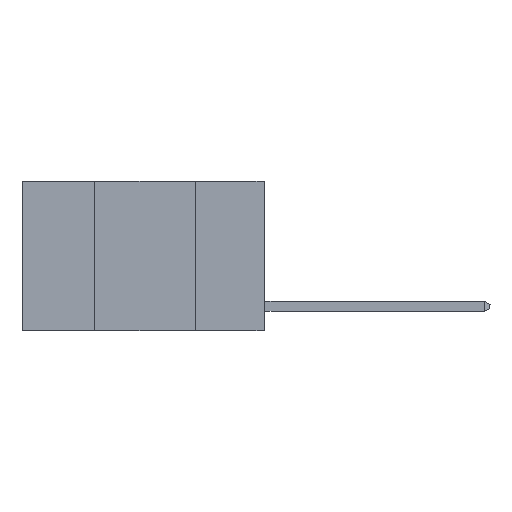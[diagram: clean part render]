
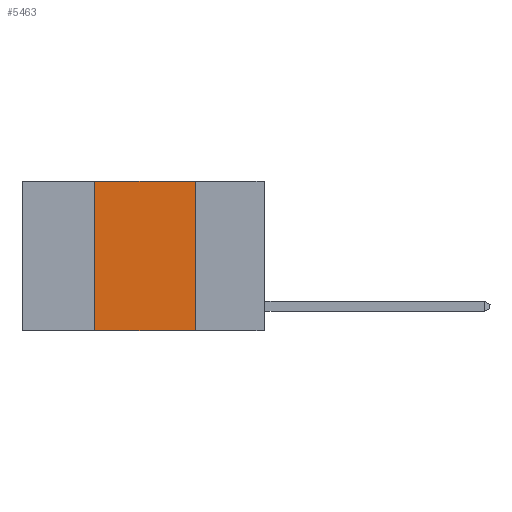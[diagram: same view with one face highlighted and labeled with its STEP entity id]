
A CAD part, left-side view. The second image highlights one B-rep face of the part: STEP entity #5463.
In plain terms, the highlighted planar face has unit normal (-1, 0, 0).
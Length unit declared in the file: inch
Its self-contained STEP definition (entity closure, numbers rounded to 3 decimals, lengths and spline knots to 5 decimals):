
#234 = LINE ( 'NONE', #14729, #4201 ) ;
#480 = AXIS2_PLACEMENT_3D ( 'NONE', #19061, #17314, #17523 ) ;
#2029 = VERTEX_POINT ( 'NONE', #8296 ) ;
#2222 = DIRECTION ( 'NONE',  ( 0., -1., 0. ) ) ;
#3056 = PLANE ( 'NONE',  #480 ) ;
#3435 = CARTESIAN_POINT ( 'NONE',  ( 0., 0.6, 0. ) ) ;
#3631 = VECTOR ( 'NONE', #7467, 39.37008 ) ;
#4201 = VECTOR ( 'NONE', #19261, 39.37008 ) ;
#4958 = EDGE_CURVE ( 'NONE', #5296, #2029, #12539, .T. ) ;
#5296 = VERTEX_POINT ( 'NONE', #13545 ) ;
#5312 = EDGE_CURVE ( 'NONE', #13542, #7009, #18152, .T. ) ;
#5463 = ADVANCED_FACE ( 'NONE', ( #18385 ), #3056, .F. ) ;
#6445 = EDGE_LOOP ( 'NONE', ( #18474, #13665, #19468, #19474 ) ) ;
#7009 = VERTEX_POINT ( 'NONE', #13013 ) ;
#7467 = DIRECTION ( 'NONE',  ( 0., 0., -1. ) ) ;
#8296 = CARTESIAN_POINT ( 'NONE',  ( 0., 0.42, 0. ) ) ;
#9358 = CARTESIAN_POINT ( 'NONE',  ( 0., 0.17, 0. ) ) ;
#10073 = EDGE_CURVE ( 'NONE', #2029, #13542, #19752, .T. ) ;
#10700 = CARTESIAN_POINT ( 'NONE',  ( 0., 0.42, 0. ) ) ;
#12539 = LINE ( 'NONE', #10700, #12769 ) ;
#12769 = VECTOR ( 'NONE', #13976, 39.37008 ) ;
#13013 = CARTESIAN_POINT ( 'NONE',  ( 0., 0.17, -0.37 ) ) ;
#13123 = VECTOR ( 'NONE', #2222, 39.37008 ) ;
#13542 = VERTEX_POINT ( 'NONE', #9358 ) ;
#13545 = CARTESIAN_POINT ( 'NONE',  ( 0., 0.42, -0.37 ) ) ;
#13665 = ORIENTED_EDGE ( 'NONE', *, *, #10073, .F. ) ;
#13976 = DIRECTION ( 'NONE',  ( 0., 0., 1. ) ) ;
#14153 = EDGE_CURVE ( 'NONE', #5296, #7009, #234, .T. ) ;
#14729 = CARTESIAN_POINT ( 'NONE',  ( 0., 0.6, -0.37 ) ) ;
#16851 = CARTESIAN_POINT ( 'NONE',  ( 0., 0.17, 0. ) ) ;
#17314 = DIRECTION ( 'NONE',  ( 1., 0., 0. ) ) ;
#17523 = DIRECTION ( 'NONE',  ( 0., 0., -1. ) ) ;
#18152 = LINE ( 'NONE', #16851, #3631 ) ;
#18385 = FACE_OUTER_BOUND ( 'NONE', #6445, .T. ) ;
#18474 = ORIENTED_EDGE ( 'NONE', *, *, #5312, .F. ) ;
#19061 = CARTESIAN_POINT ( 'NONE',  ( 0., 0.6, 0. ) ) ;
#19261 = DIRECTION ( 'NONE',  ( 0., -1., 0. ) ) ;
#19468 = ORIENTED_EDGE ( 'NONE', *, *, #4958, .F. ) ;
#19474 = ORIENTED_EDGE ( 'NONE', *, *, #14153, .T. ) ;
#19752 = LINE ( 'NONE', #3435, #13123 ) ;
